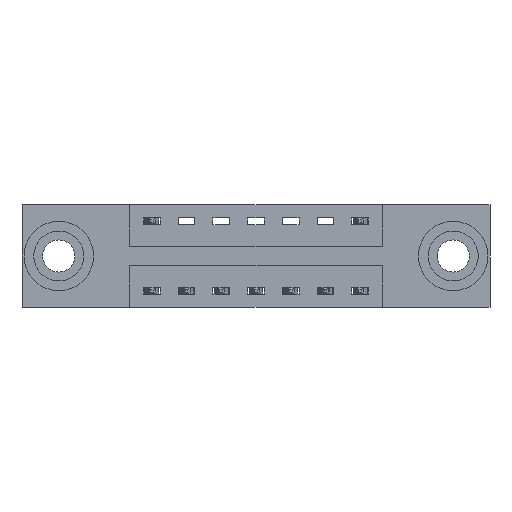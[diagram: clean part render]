
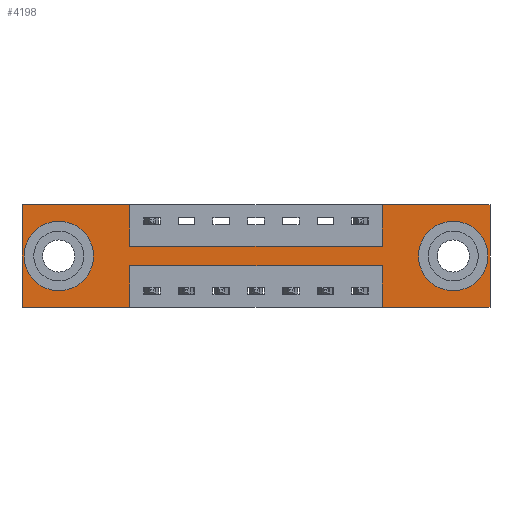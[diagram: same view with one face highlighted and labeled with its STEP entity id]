
A CAD part, front view. The second image highlights one B-rep face of the part: STEP entity #4198.
In plain terms, the highlighted planar face has unit normal (0, -1, 0).
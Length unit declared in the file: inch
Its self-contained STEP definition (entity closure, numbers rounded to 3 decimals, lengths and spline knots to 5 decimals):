
#32 = ORIENTED_EDGE ( 'NONE', *, *, #8464, .F. ) ;
#72 = VECTOR ( 'NONE', #2180, 39.37008 ) ;
#87 = CARTESIAN_POINT ( 'NONE',  ( 0., 0., 0. ) ) ;
#115 = ORIENTED_EDGE ( 'NONE', *, *, #8669, .F. ) ;
#125 = VERTEX_POINT ( 'NONE', #7183 ) ;
#138 = EDGE_LOOP ( 'NONE', ( #8285, #5339, #502, #2761, #870, #5853, #7707, #7478, #115, #6923, #1666, #32 ) ) ;
#147 = CARTESIAN_POINT ( 'NONE',  ( 0., 0., -0.37 ) ) ;
#170 = VERTEX_POINT ( 'NONE', #6041 ) ;
#271 = CARTESIAN_POINT ( 'NONE',  ( 0.3875, 0., -0.22 ) ) ;
#306 = ORIENTED_EDGE ( 'NONE', *, *, #4309, .T. ) ;
#360 = VERTEX_POINT ( 'NONE', #6737 ) ;
#435 = CARTESIAN_POINT ( 'NONE',  ( 1.685, 0., -0.37 ) ) ;
#502 = ORIENTED_EDGE ( 'NONE', *, *, #8156, .F. ) ;
#573 = FACE_BOUND ( 'NONE', #8089, .T. ) ;
#714 = AXIS2_PLACEMENT_3D ( 'NONE', #7913, #8616, #4062 ) ;
#791 = VECTOR ( 'NONE', #6084, 39.37008 ) ;
#870 = ORIENTED_EDGE ( 'NONE', *, *, #5357, .F. ) ;
#954 = DIRECTION ( 'NONE',  ( 1., 0., 0. ) ) ;
#1109 = LINE ( 'NONE', #8983, #5356 ) ;
#1208 = VERTEX_POINT ( 'NONE', #7082 ) ;
#1385 = AXIS2_PLACEMENT_3D ( 'NONE', #3445, #8746, #4224 ) ;
#1396 = CARTESIAN_POINT ( 'NONE',  ( 0.1325, 0., -0.107 ) ) ;
#1420 = CARTESIAN_POINT ( 'NONE',  ( 0.3875, 0., -0.15 ) ) ;
#1529 = LINE ( 'NONE', #2810, #7756 ) ;
#1637 = CIRCLE ( 'NONE', #2519, 0.078 ) ;
#1662 = CARTESIAN_POINT ( 'NONE',  ( 0.1325, 0., -0.185 ) ) ;
#1666 = ORIENTED_EDGE ( 'NONE', *, *, #5046, .F. ) ;
#1695 = CARTESIAN_POINT ( 'NONE',  ( 0., 0., 0. ) ) ;
#1928 = VERTEX_POINT ( 'NONE', #3174 ) ;
#2102 = VERTEX_POINT ( 'NONE', #87 ) ;
#2180 = DIRECTION ( 'NONE',  ( 1., 0., 0. ) ) ;
#2378 = LINE ( 'NONE', #1420, #72 ) ;
#2458 = PLANE ( 'NONE',  #714 ) ;
#2465 = DIRECTION ( 'NONE',  ( 0., 0., 1. ) ) ;
#2519 = AXIS2_PLACEMENT_3D ( 'NONE', #3859, #9115, #4650 ) ;
#2543 = CARTESIAN_POINT ( 'NONE',  ( 1.685, 0., 0. ) ) ;
#2604 = CARTESIAN_POINT ( 'NONE',  ( 0.3875, 0., -0.37 ) ) ;
#2625 = CARTESIAN_POINT ( 'NONE',  ( 0.3875, 0., -0.37 ) ) ;
#2637 = DIRECTION ( 'NONE',  ( -1., 0., 0. ) ) ;
#2683 = DIRECTION ( 'NONE',  ( 0., 1., 0. ) ) ;
#2761 = ORIENTED_EDGE ( 'NONE', *, *, #8997, .F. ) ;
#2810 = CARTESIAN_POINT ( 'NONE',  ( 1.2975, 0., -0.37 ) ) ;
#3017 = VECTOR ( 'NONE', #3850, 39.37008 ) ;
#3041 = VERTEX_POINT ( 'NONE', #435 ) ;
#3065 = CIRCLE ( 'NONE', #3903, 0.078 ) ;
#3174 = CARTESIAN_POINT ( 'NONE',  ( 1.5525, 0., -0.107 ) ) ;
#3445 = CARTESIAN_POINT ( 'NONE',  ( 1.5525, 0., -0.185 ) ) ;
#3661 = CARTESIAN_POINT ( 'NONE',  ( 1.5525, 0., -0.263 ) ) ;
#3677 = VECTOR ( 'NONE', #5045, 39.37008 ) ;
#3850 = DIRECTION ( 'NONE',  ( 1., 0., 0. ) ) ;
#3859 = CARTESIAN_POINT ( 'NONE',  ( 0.1325, 0., -0.185 ) ) ;
#3903 = AXIS2_PLACEMENT_3D ( 'NONE', #7364, #2683, #8098 ) ;
#4062 = DIRECTION ( 'NONE',  ( 0., 0., -1. ) ) ;
#4198 = ADVANCED_FACE ( 'NONE', ( #8570, #573, #4802 ), #2458, .T. ) ;
#4224 = DIRECTION ( 'NONE',  ( 0., 0., -1. ) ) ;
#4285 = ORIENTED_EDGE ( 'NONE', *, *, #4872, .T. ) ;
#4309 = EDGE_CURVE ( 'NONE', #7181, #1928, #3065, .T. ) ;
#4525 = VERTEX_POINT ( 'NONE', #1396 ) ;
#4650 = DIRECTION ( 'NONE',  ( 0., 0., 1. ) ) ;
#4676 = CARTESIAN_POINT ( 'NONE',  ( 0.3875, 0., -0.22 ) ) ;
#4754 = DIRECTION ( 'NONE',  ( -1., 0., 0. ) ) ;
#4802 = FACE_OUTER_BOUND ( 'NONE', #138, .T. ) ;
#4824 = VECTOR ( 'NONE', #954, 39.37008 ) ;
#4838 = VERTEX_POINT ( 'NONE', #8685 ) ;
#4872 = EDGE_CURVE ( 'NONE', #1928, #7181, #7321, .T. ) ;
#5045 = DIRECTION ( 'NONE',  ( 0., 0., -1. ) ) ;
#5046 = EDGE_CURVE ( 'NONE', #170, #2102, #1109, .T. ) ;
#5107 = VERTEX_POINT ( 'NONE', #8362 ) ;
#5142 = VECTOR ( 'NONE', #4754, 39.37008 ) ;
#5161 = VERTEX_POINT ( 'NONE', #4676 ) ;
#5217 = VERTEX_POINT ( 'NONE', #6303 ) ;
#5270 = CARTESIAN_POINT ( 'NONE',  ( 1.685, 0., 0. ) ) ;
#5339 = ORIENTED_EDGE ( 'NONE', *, *, #8121, .F. ) ;
#5356 = VECTOR ( 'NONE', #9638, 39.37008 ) ;
#5357 = EDGE_CURVE ( 'NONE', #5951, #3041, #7588, .T. ) ;
#5382 = LINE ( 'NONE', #9103, #3017 ) ;
#5410 = VERTEX_POINT ( 'NONE', #2625 ) ;
#5534 = LINE ( 'NONE', #9624, #791 ) ;
#5577 = CARTESIAN_POINT ( 'NONE',  ( 0., 0., -0.37 ) ) ;
#5719 = EDGE_CURVE ( 'NONE', #2102, #4838, #7357, .T. ) ;
#5776 = VECTOR ( 'NONE', #5883, 39.37008 ) ;
#5786 = LINE ( 'NONE', #2604, #3677 ) ;
#5853 = ORIENTED_EDGE ( 'NONE', *, *, #8930, .F. ) ;
#5883 = DIRECTION ( 'NONE',  ( 0., 0., -1. ) ) ;
#5951 = VERTEX_POINT ( 'NONE', #5270 ) ;
#6017 = LINE ( 'NONE', #271, #9588 ) ;
#6041 = CARTESIAN_POINT ( 'NONE',  ( 0., 0., -0.37 ) ) ;
#6084 = DIRECTION ( 'NONE',  ( 0., 0., 1. ) ) ;
#6303 = CARTESIAN_POINT ( 'NONE',  ( 0.3875, 0., -0.15 ) ) ;
#6475 = LINE ( 'NONE', #147, #8202 ) ;
#6732 = DIRECTION ( 'NONE',  ( 0., 0., 1. ) ) ;
#6737 = CARTESIAN_POINT ( 'NONE',  ( 1.2975, 0., -0.22 ) ) ;
#6923 = ORIENTED_EDGE ( 'NONE', *, *, #5719, .F. ) ;
#6982 = VERTEX_POINT ( 'NONE', #7896 ) ;
#7082 = CARTESIAN_POINT ( 'NONE',  ( 1.2975, 0., 0. ) ) ;
#7163 = DIRECTION ( 'NONE',  ( 0., 1., 0. ) ) ;
#7181 = VERTEX_POINT ( 'NONE', #3661 ) ;
#7183 = CARTESIAN_POINT ( 'NONE',  ( 1.2975, 0., -0.15 ) ) ;
#7321 = CIRCLE ( 'NONE', #1385, 0.078 ) ;
#7357 = LINE ( 'NONE', #1695, #4824 ) ;
#7364 = CARTESIAN_POINT ( 'NONE',  ( 1.5525, 0., -0.185 ) ) ;
#7385 = AXIS2_PLACEMENT_3D ( 'NONE', #1662, #7163, #2465 ) ;
#7478 = ORIENTED_EDGE ( 'NONE', *, *, #8288, .F. ) ;
#7588 = LINE ( 'NONE', #2543, #9449 ) ;
#7707 = ORIENTED_EDGE ( 'NONE', *, *, #8217, .F. ) ;
#7756 = VECTOR ( 'NONE', #6732, 39.37008 ) ;
#7767 = ORIENTED_EDGE ( 'NONE', *, *, #8971, .T. ) ;
#7817 = ORIENTED_EDGE ( 'NONE', *, *, #8312, .T. ) ;
#7896 = CARTESIAN_POINT ( 'NONE',  ( 0.1325, 0., -0.263 ) ) ;
#7913 = CARTESIAN_POINT ( 'NONE',  ( 0., 0., -0.37 ) ) ;
#7989 = DIRECTION ( 'NONE',  ( 0., 0., -1. ) ) ;
#8089 = EDGE_LOOP ( 'NONE', ( #7817, #7767 ) ) ;
#8098 = DIRECTION ( 'NONE',  ( 0., 0., -1. ) ) ;
#8121 = EDGE_CURVE ( 'NONE', #360, #5161, #6017, .T. ) ;
#8131 = EDGE_CURVE ( 'NONE', #5161, #5410, #5786, .T. ) ;
#8156 = EDGE_CURVE ( 'NONE', #5107, #360, #1529, .T. ) ;
#8202 = VECTOR ( 'NONE', #9286, 39.37008 ) ;
#8217 = EDGE_CURVE ( 'NONE', #125, #1208, #5534, .T. ) ;
#8285 = ORIENTED_EDGE ( 'NONE', *, *, #8131, .F. ) ;
#8288 = EDGE_CURVE ( 'NONE', #5217, #125, #2378, .T. ) ;
#8305 = EDGE_LOOP ( 'NONE', ( #4285, #306 ) ) ;
#8312 = EDGE_CURVE ( 'NONE', #4525, #6982, #1637, .T. ) ;
#8362 = CARTESIAN_POINT ( 'NONE',  ( 1.2975, 0., -0.37 ) ) ;
#8464 = EDGE_CURVE ( 'NONE', #5410, #170, #9070, .T. ) ;
#8570 = FACE_BOUND ( 'NONE', #8305, .T. ) ;
#8616 = DIRECTION ( 'NONE',  ( 0., -1., 0. ) ) ;
#8669 = EDGE_CURVE ( 'NONE', #4838, #5217, #9773, .T. ) ;
#8685 = CARTESIAN_POINT ( 'NONE',  ( 0.3875, 0., 0. ) ) ;
#8746 = DIRECTION ( 'NONE',  ( 0., 1., 0. ) ) ;
#8796 = CARTESIAN_POINT ( 'NONE',  ( 0.3875, 0., 0. ) ) ;
#8836 = CIRCLE ( 'NONE', #7385, 0.078 ) ;
#8930 = EDGE_CURVE ( 'NONE', #1208, #5951, #5382, .T. ) ;
#8971 = EDGE_CURVE ( 'NONE', #6982, #4525, #8836, .T. ) ;
#8983 = CARTESIAN_POINT ( 'NONE',  ( 0., 0., 0. ) ) ;
#8997 = EDGE_CURVE ( 'NONE', #3041, #5107, #6475, .T. ) ;
#9070 = LINE ( 'NONE', #5577, #5142 ) ;
#9103 = CARTESIAN_POINT ( 'NONE',  ( 0., 0., 0. ) ) ;
#9115 = DIRECTION ( 'NONE',  ( 0., 1., 0. ) ) ;
#9286 = DIRECTION ( 'NONE',  ( -1., 0., 0. ) ) ;
#9449 = VECTOR ( 'NONE', #7989, 39.37008 ) ;
#9588 = VECTOR ( 'NONE', #2637, 39.37008 ) ;
#9624 = CARTESIAN_POINT ( 'NONE',  ( 1.2975, 0., 0. ) ) ;
#9638 = DIRECTION ( 'NONE',  ( 0., 0., 1. ) ) ;
#9773 = LINE ( 'NONE', #8796, #5776 ) ;
